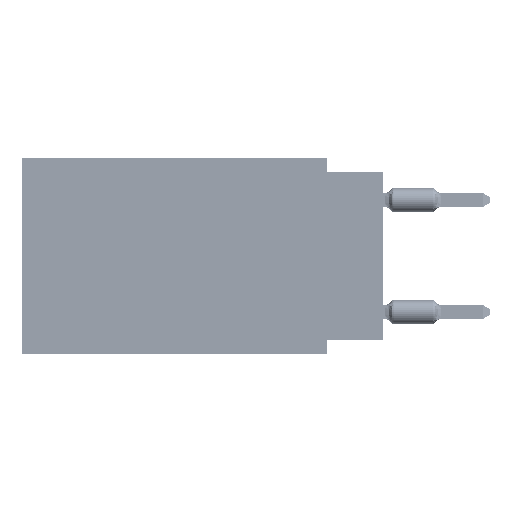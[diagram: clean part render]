
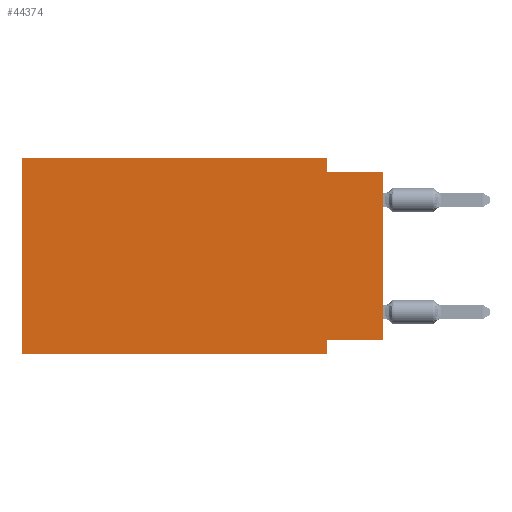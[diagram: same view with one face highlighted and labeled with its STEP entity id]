
A CAD part, left-side view. The second image highlights one B-rep face of the part: STEP entity #44374.
In plain terms, the highlighted planar face has unit normal (-1, 0, 0).
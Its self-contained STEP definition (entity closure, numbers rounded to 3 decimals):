
#1085 = CARTESIAN_POINT ( 'NONE',  ( 0., 16.383, -8.89 ) ) ;
#1678 = LINE ( 'NONE', #84361, #21534 ) ;
#1938 = CARTESIAN_POINT ( 'NONE',  ( 0., 16.383, 0. ) ) ;
#4285 = EDGE_CURVE ( 'NONE', #15140, #23107, #90676, .T. ) ;
#4343 = ORIENTED_EDGE ( 'NONE', *, *, #104296, .F. ) ;
#7109 = LINE ( 'NONE', #78881, #31926 ) ;
#9239 = VERTEX_POINT ( 'NONE', #59613 ) ;
#10211 = DIRECTION ( 'NONE',  ( 0., -1., 0. ) ) ;
#11097 = ORIENTED_EDGE ( 'NONE', *, *, #110266, .T. ) ;
#13725 = VECTOR ( 'NONE', #119850, 1000. ) ;
#15140 = VERTEX_POINT ( 'NONE', #110942 ) ;
#16841 = ORIENTED_EDGE ( 'NONE', *, *, #33898, .F. ) ;
#17417 = EDGE_CURVE ( 'NONE', #78497, #9239, #61929, .T. ) ;
#19647 = DIRECTION ( 'NONE',  ( 0., 0., 1. ) ) ;
#20772 = DIRECTION ( 'NONE',  ( 0., 0., -1. ) ) ;
#21534 = VECTOR ( 'NONE', #77633, 1000. ) ;
#23107 = VERTEX_POINT ( 'NONE', #79737 ) ;
#23197 = VECTOR ( 'NONE', #19647, 1000. ) ;
#26573 = EDGE_CURVE ( 'NONE', #99641, #9239, #56402, .T. ) ;
#31926 = VECTOR ( 'NONE', #33313, 1000. ) ;
#32032 = ORIENTED_EDGE ( 'NONE', *, *, #17417, .F. ) ;
#33313 = DIRECTION ( 'NONE',  ( 0., -1., 0. ) ) ;
#33816 = DIRECTION ( 'NONE',  ( 0., 0., 1. ) ) ;
#33898 = EDGE_CURVE ( 'NONE', #76799, #112494, #7109, .T. ) ;
#39023 = DIRECTION ( 'NONE',  ( 1., 0., 0. ) ) ;
#43756 = ORIENTED_EDGE ( 'NONE', *, *, #61494, .F. ) ;
#44374 = ADVANCED_FACE ( 'NONE', ( #48134 ), #85227, .F. ) ;
#46342 = EDGE_LOOP ( 'NONE', ( #11097, #71104, #4343, #16841, #97480, #65159, #32032, #43756 ) ) ;
#47600 = LINE ( 'NONE', #95622, #23197 ) ;
#48134 = FACE_OUTER_BOUND ( 'NONE', #46342, .T. ) ;
#53831 = LINE ( 'NONE', #61164, #77988 ) ;
#56402 = LINE ( 'NONE', #1085, #110656 ) ;
#57143 = LINE ( 'NONE', #65062, #96455 ) ;
#57613 = CARTESIAN_POINT ( 'NONE',  ( 0., 0., -8.255 ) ) ;
#57708 = VECTOR ( 'NONE', #89308, 1000. ) ;
#59031 = EDGE_CURVE ( 'NONE', #99641, #76799, #47600, .T. ) ;
#59613 = CARTESIAN_POINT ( 'NONE',  ( 0., 2.54, -8.89 ) ) ;
#61164 = CARTESIAN_POINT ( 'NONE',  ( 0., 0., 0. ) ) ;
#61494 = EDGE_CURVE ( 'NONE', #110660, #78497, #1678, .T. ) ;
#61929 = LINE ( 'NONE', #116084, #57708 ) ;
#62140 = CARTESIAN_POINT ( 'NONE',  ( 0., 16.383, 0. ) ) ;
#65062 = CARTESIAN_POINT ( 'NONE',  ( 0., 2.54, 0. ) ) ;
#65159 = ORIENTED_EDGE ( 'NONE', *, *, #26573, .T. ) ;
#68986 = CARTESIAN_POINT ( 'NONE',  ( 0., 2.54, 0. ) ) ;
#71104 = ORIENTED_EDGE ( 'NONE', *, *, #4285, .F. ) ;
#76799 = VERTEX_POINT ( 'NONE', #62140 ) ;
#77633 = DIRECTION ( 'NONE',  ( 0., 1., 0. ) ) ;
#77988 = VECTOR ( 'NONE', #33816, 1000. ) ;
#78497 = VERTEX_POINT ( 'NONE', #113768 ) ;
#78881 = CARTESIAN_POINT ( 'NONE',  ( 0., 16.383, 0. ) ) ;
#79308 = AXIS2_PLACEMENT_3D ( 'NONE', #1938, #39023, #20772 ) ;
#79737 = CARTESIAN_POINT ( 'NONE',  ( 0., 0., -0.635 ) ) ;
#80514 = CARTESIAN_POINT ( 'NONE',  ( 0., 16.383, -8.89 ) ) ;
#82748 = CARTESIAN_POINT ( 'NONE',  ( 0., 0., -0.635 ) ) ;
#84361 = CARTESIAN_POINT ( 'NONE',  ( 0., 0., -8.255 ) ) ;
#85227 = PLANE ( 'NONE',  #79308 ) ;
#89308 = DIRECTION ( 'NONE',  ( 0., 0., -1. ) ) ;
#90676 = LINE ( 'NONE', #82748, #13725 ) ;
#94238 = DIRECTION ( 'NONE',  ( 0., 0., -1. ) ) ;
#95622 = CARTESIAN_POINT ( 'NONE',  ( 0., 16.383, 0. ) ) ;
#96455 = VECTOR ( 'NONE', #94238, 1000. ) ;
#97480 = ORIENTED_EDGE ( 'NONE', *, *, #59031, .F. ) ;
#99641 = VERTEX_POINT ( 'NONE', #80514 ) ;
#104296 = EDGE_CURVE ( 'NONE', #112494, #15140, #57143, .T. ) ;
#110266 = EDGE_CURVE ( 'NONE', #110660, #23107, #53831, .T. ) ;
#110656 = VECTOR ( 'NONE', #10211, 1000. ) ;
#110660 = VERTEX_POINT ( 'NONE', #57613 ) ;
#110942 = CARTESIAN_POINT ( 'NONE',  ( 0., 2.54, -0.635 ) ) ;
#112494 = VERTEX_POINT ( 'NONE', #68986 ) ;
#113768 = CARTESIAN_POINT ( 'NONE',  ( 0., 2.54, -8.255 ) ) ;
#116084 = CARTESIAN_POINT ( 'NONE',  ( 0., 2.54, -8.89 ) ) ;
#119850 = DIRECTION ( 'NONE',  ( 0., -1., 0. ) ) ;
